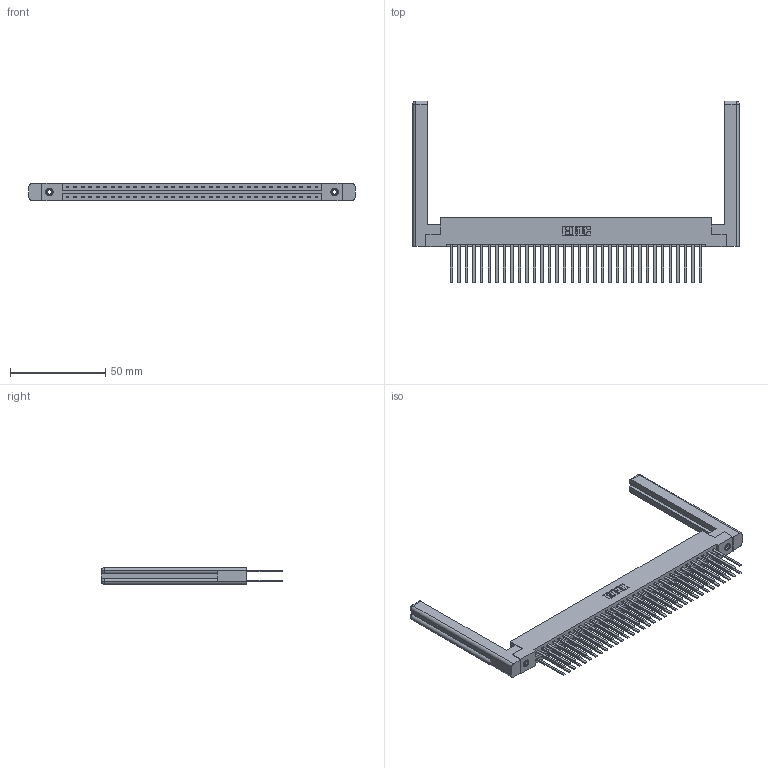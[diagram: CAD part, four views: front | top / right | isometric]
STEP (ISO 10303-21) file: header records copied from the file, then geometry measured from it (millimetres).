
FILE_DESCRIPTION (( 'STEP AP203' ), '1' );
FILE_NAME ('337-068-544-258.STEP', '2019-10-10T00:28:19', ( '' ), ( '' ), 'SwSTEP 2.0', 'SolidWorks 2016', '' );
FILE_SCHEMA (( 'CONFIG_CONTROL_DESIGN' ));
Length unit declared in the file: inch
Products named in the file (5): 307-220-058; 337-068-544-258; 337 Part_Flush Mounting Lugs - 0.156 Dia-TI; 345-250-001_345-250-001-102; 345-292-001_345-293-144
Assembly tree (73 placements, depth 2):
  337-068-544-258
    337 Part_Flush Mounting Lugs - 0.156 Dia-TI
    345-292-001_345-293-144  x68
    345-250-001_345-250-001-102  x2
    307-220-058  x2
Bounding box: 171.35 x 95.38 x 9.4 mm (x, y, z)
Volume: 26047.1 mm3; surface area: 29454.9 mm2
Topology: 73 solids, 73 shells, 3520 faces, 10389 edges, 6822 vertices
Faces by surface type: plane 2466, cylinder 1030, cone 12, torus 12
Entity records: 29846 total; most frequent: CARTESIAN_POINT 5041, ORIENTED_EDGE 4916, DIRECTION 4314, EDGE_CURVE 2458, VECTOR 2286, LINE 2286, VERTEX_POINT 1630, AXIS2_PLACEMENT_3D 1014
